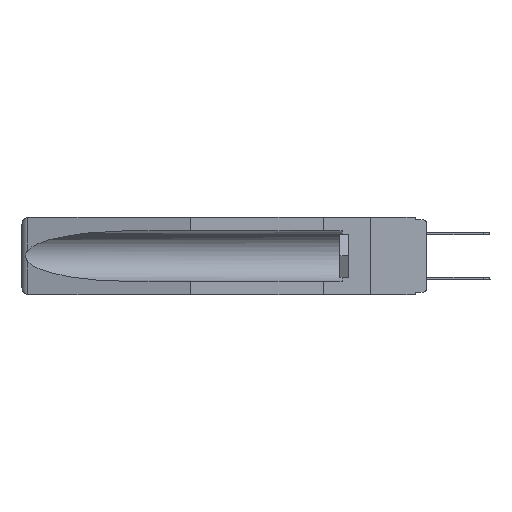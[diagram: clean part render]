
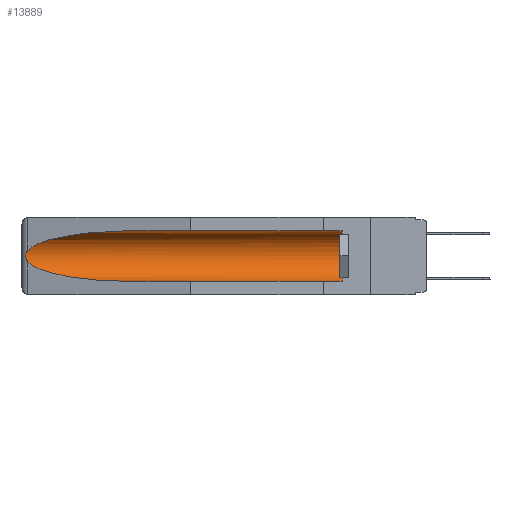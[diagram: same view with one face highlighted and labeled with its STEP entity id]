
A CAD part, left-side view. The second image highlights one B-rep face of the part: STEP entity #13889.
In plain terms, the highlighted cylindrical face has radius 2.857 mm (diameter 5.715 mm), a partial arc.
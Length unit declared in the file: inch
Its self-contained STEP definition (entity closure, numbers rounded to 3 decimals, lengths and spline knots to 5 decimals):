
#327 = VECTOR ( 'NONE', #24341, 39.37008 ) ;
#409 = CIRCLE ( 'NONE', #16173, 0.1125 ) ;
#461 = ORIENTED_EDGE ( 'NONE', *, *, #21803, .T. ) ;
#820 = CARTESIAN_POINT ( 'NONE',  ( 0.25451, 1.48313, -0.24835 ) ) ;
#899 = DIRECTION ( 'NONE',  ( 0., 1., 0. ) ) ;
#1092 = CARTESIAN_POINT ( 'NONE',  ( 0.155, 0.126, -0.284 ) ) ;
#1368 = CARTESIAN_POINT ( 'NONE',  ( 0.2673, 1.5327, -0.16383 ) ) ;
#1704 = ORIENTED_EDGE ( 'NONE', *, *, #17776, .T. ) ;
#1881 = DIRECTION ( 'NONE',  ( 0., 0., 1. ) ) ;
#2742 = CARTESIAN_POINT ( 'NONE',  ( 0.21114, 1.30732, -0.059 ) ) ;
#2767 = DIRECTION ( 'NONE',  ( 0., 0., 1. ) ) ;
#3008 = VERTEX_POINT ( 'NONE', #1092 ) ;
#3481 = CARTESIAN_POINT ( 'NONE',  ( 0.26537, 1.52718, -0.14972 ) ) ;
#4279 = CARTESIAN_POINT ( 'NONE',  ( 0.155, 0.126, -0.059 ) ) ;
#5433 = CARTESIAN_POINT ( 'NONE',  ( 0.2675, 1.53308, -0.16763 ) ) ;
#6316 = VERTEX_POINT ( 'NONE', #13803 ) ;
#6519 = CARTESIAN_POINT ( 'NONE',  ( 0.26537, 1.52718, -0.19328 ) ) ;
#6631 = CARTESIAN_POINT ( 'NONE',  ( 0.155, 1.07973, -0.059 ) ) ;
#7463 = CARTESIAN_POINT ( 'NONE',  ( 0.2673, 1.53269, -0.17917 ) ) ;
#7623 = B_SPLINE_CURVE_WITH_KNOTS ( 'NONE', 3,
 ( #3481, #19551, #15366, #1368, #5433, #19474, #7463, #21493, #9485, #23503 ),
 .UNSPECIFIED., .F., .F.,
 ( 4, 2, 2, 2, 4 ),
 ( 0., 0.00029, 0.00058, 0.00087, 0.00117 ),
 .UNSPECIFIED. ) ;
#8510 = EDGE_LOOP ( 'NONE', ( #461, #13958, #16307, #24704, #1704, #20982 ) ) ;
#9485 = CARTESIAN_POINT ( 'NONE',  ( 0.26597, 1.5296, -0.19026 ) ) ;
#10284 = VERTEX_POINT ( 'NONE', #21511 ) ;
#11151 =( BOUNDED_CURVE ( )  B_SPLINE_CURVE ( 3, ( #6631, #2742, #14533, #12758 ),
 .UNSPECIFIED., .F., .T. ) 
 B_SPLINE_CURVE_WITH_KNOTS ( ( 4, 4 ),
 ( 4.71239, 6.08839 ),
 .UNSPECIFIED. ) 
 CURVE ( )  GEOMETRIC_REPRESENTATION_ITEM ( )  RATIONAL_B_SPLINE_CURVE ( ( 1., 0.848, 0.848, 1. ) ) 
 REPRESENTATION_ITEM ( '' )  );
#11922 = DIRECTION ( 'NONE',  ( 0., -1., 0. ) ) ;
#12127 = CARTESIAN_POINT ( 'NONE',  ( 0.26537, 1.52718, -0.14972 ) ) ;
#12291 = CARTESIAN_POINT ( 'NONE',  ( 0.155, -0.30754, -0.284 ) ) ;
#12758 = CARTESIAN_POINT ( 'NONE',  ( 0.26537, 1.52718, -0.14972 ) ) ;
#12970 = CARTESIAN_POINT ( 'NONE',  ( 0.21114, 1.30732, -0.284 ) ) ;
#13204 = FACE_OUTER_BOUND ( 'NONE', #8510, .T. ) ;
#13803 = CARTESIAN_POINT ( 'NONE',  ( 0.155, 1.07973, -0.059 ) ) ;
#13889 = ADVANCED_FACE ( 'NONE', ( #13204 ), #21673, .F. ) ;
#13958 = ORIENTED_EDGE ( 'NONE', *, *, #17673, .T. ) ;
#14533 = CARTESIAN_POINT ( 'NONE',  ( 0.25451, 1.48313, -0.09465 ) ) ;
#14824 = CARTESIAN_POINT ( 'NONE',  ( 0.155, -0.30754, -0.1715 ) ) ;
#14904 = VERTEX_POINT ( 'NONE', #4279 ) ;
#15366 = CARTESIAN_POINT ( 'NONE',  ( 0.26654, 1.53092, -0.15636 ) ) ;
#15604 = CARTESIAN_POINT ( 'NONE',  ( 0.155, 0.126, -0.1715 ) ) ;
#16173 = AXIS2_PLACEMENT_3D ( 'NONE', #15604, #11922, #1881 ) ;
#16296 = CARTESIAN_POINT ( 'NONE',  ( 0.155, -0.30754, -0.059 ) ) ;
#16307 = ORIENTED_EDGE ( 'NONE', *, *, #24219, .T. ) ;
#16582 = VECTOR ( 'NONE', #18579, 39.37008 ) ;
#17673 = EDGE_CURVE ( 'NONE', #24060, #24816, #7623, .T. ) ;
#17776 = EDGE_CURVE ( 'NONE', #3008, #14904, #409, .T. ) ;
#18203 =( BOUNDED_CURVE ( )  B_SPLINE_CURVE ( 3, ( #22855, #820, #12970, #21033 ),
 .UNSPECIFIED., .F., .F. ) 
 B_SPLINE_CURVE_WITH_KNOTS ( ( 4, 4 ),
 ( 0.1948, 1.5708 ),
 .UNSPECIFIED. ) 
 CURVE ( )  GEOMETRIC_REPRESENTATION_ITEM ( )  RATIONAL_B_SPLINE_CURVE ( ( 1., 0.848, 0.848, 1. ) ) 
 REPRESENTATION_ITEM ( '' )  );
#18363 = EDGE_CURVE ( 'NONE', #14904, #6316, #18879, .T. ) ;
#18579 = DIRECTION ( 'NONE',  ( 0., 1., 0. ) ) ;
#18879 = LINE ( 'NONE', #16296, #327 ) ;
#19474 = CARTESIAN_POINT ( 'NONE',  ( 0.2675, 1.53308, -0.17534 ) ) ;
#19551 = CARTESIAN_POINT ( 'NONE',  ( 0.26597, 1.52961, -0.15275 ) ) ;
#20835 = AXIS2_PLACEMENT_3D ( 'NONE', #14824, #899, #2767 ) ;
#20982 = ORIENTED_EDGE ( 'NONE', *, *, #18363, .T. ) ;
#21033 = CARTESIAN_POINT ( 'NONE',  ( 0.155, 1.07973, -0.284 ) ) ;
#21493 = CARTESIAN_POINT ( 'NONE',  ( 0.26655, 1.53094, -0.18657 ) ) ;
#21511 = CARTESIAN_POINT ( 'NONE',  ( 0.155, 1.07973, -0.284 ) ) ;
#21673 = CYLINDRICAL_SURFACE ( 'NONE', #20835, 0.1125 ) ;
#21803 = EDGE_CURVE ( 'NONE', #6316, #24060, #11151, .T. ) ;
#22429 = EDGE_CURVE ( 'NONE', #3008, #10284, #25695, .T. ) ;
#22855 = CARTESIAN_POINT ( 'NONE',  ( 0.26537, 1.52718, -0.19328 ) ) ;
#23503 = CARTESIAN_POINT ( 'NONE',  ( 0.26537, 1.52718, -0.19328 ) ) ;
#24060 = VERTEX_POINT ( 'NONE', #12127 ) ;
#24219 = EDGE_CURVE ( 'NONE', #24816, #10284, #18203, .T. ) ;
#24341 = DIRECTION ( 'NONE',  ( 0., 1., 0. ) ) ;
#24704 = ORIENTED_EDGE ( 'NONE', *, *, #22429, .F. ) ;
#24816 = VERTEX_POINT ( 'NONE', #6519 ) ;
#25695 = LINE ( 'NONE', #12291, #16582 ) ;
